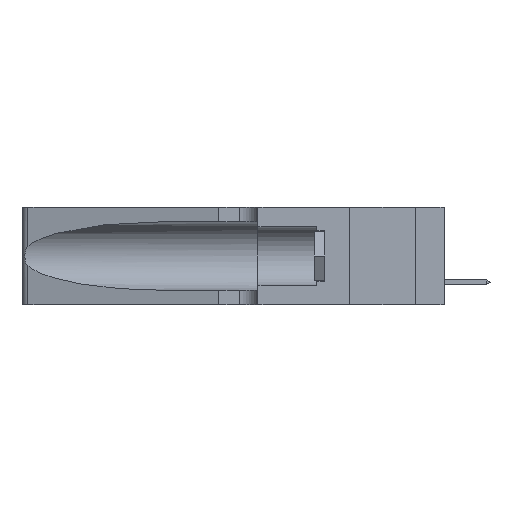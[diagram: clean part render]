
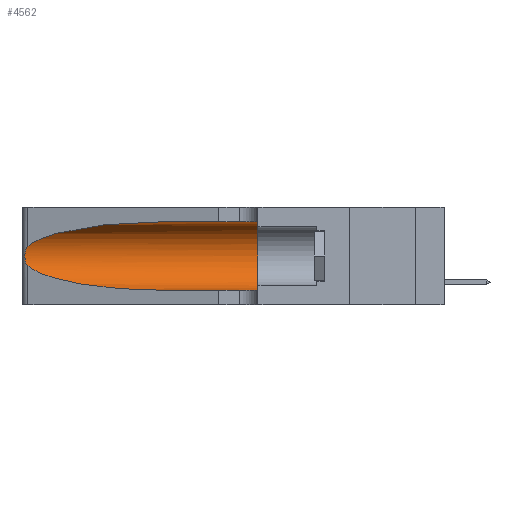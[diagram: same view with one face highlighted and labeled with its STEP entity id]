
A CAD part, left-side view. The second image highlights one B-rep face of the part: STEP entity #4562.
In plain terms, the highlighted cylindrical face has radius 3.308 mm (diameter 6.617 mm), a partial arc.
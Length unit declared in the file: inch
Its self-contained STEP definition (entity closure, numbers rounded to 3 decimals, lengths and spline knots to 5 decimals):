
#652 = ORIENTED_EDGE ( 'NONE', *, *, #2996, .T. ) ;
#732 = LINE ( 'NONE', #8319, #9041 ) ;
#810 = EDGE_CURVE ( 'NONE', #3578, #13876, #20713, .T. ) ;
#1320 = DIRECTION ( 'NONE',  ( 0., -1., 0. ) ) ;
#1376 = CARTESIAN_POINT ( 'NONE',  ( 0.25639, 1.23184, 0.21858 ) ) ;
#1530 = CARTESIAN_POINT ( 'NONE',  ( 0.25789, 1.23486, 0.15765 ) ) ;
#2424 =( BOUNDED_CURVE ( )  B_SPLINE_CURVE ( 3, ( #16132, #9029, #17956, #18024 ),
 .UNSPECIFIED., .F., .F. ) 
 B_SPLINE_CURVE_WITH_KNOTS ( ( 4, 4 ),
 ( 3.44316, 4.71239 ),
 .UNSPECIFIED. ) 
 CURVE ( )  GEOMETRIC_REPRESENTATION_ITEM ( )  RATIONAL_B_SPLINE_CURVE ( ( 1., 0.87, 0.87, 1. ) ) 
 REPRESENTATION_ITEM ( '' )  );
#2996 = EDGE_CURVE ( 'NONE', #15534, #13876, #9324, .T. ) ;
#3229 = CARTESIAN_POINT ( 'NONE',  ( 0.25854, 1.2359, 0.20912 ) ) ;
#3366 = DIRECTION ( 'NONE',  ( 0., -1., 0. ) ) ;
#3578 = VERTEX_POINT ( 'NONE', #5472 ) ;
#4065 = CARTESIAN_POINT ( 'NONE',  ( 0.18966, 0.96281, 0.31525 ) ) ;
#4504 = VECTOR ( 'NONE', #1320, 39.37008 ) ;
#4562 = ADVANCED_FACE ( 'NONE', ( #17464 ), #7822, .F. ) ;
#4864 = EDGE_LOOP ( 'NONE', ( #17636, #15451, #6597, #652, #12323, #9043 ) ) ;
#4924 = CARTESIAN_POINT ( 'NONE',  ( 0.25487, 1.22718, 0.22369 ) ) ;
#5076 = CARTESIAN_POINT ( 'NONE',  ( 0.26075, 1.23896, 0.19203 ) ) ;
#5120 = DIRECTION ( 'NONE',  ( 0., 0., -1. ) ) ;
#5224 = CARTESIAN_POINT ( 'NONE',  ( 0.26018, 1.23835, 0.19895 ) ) ;
#5472 = CARTESIAN_POINT ( 'NONE',  ( 0.1305, 0.35, 0.31525 ) ) ;
#6391 = CARTESIAN_POINT ( 'NONE',  ( 0.1305, 0.72297, 0.05475 ) ) ;
#6597 = ORIENTED_EDGE ( 'NONE', *, *, #18914, .T. ) ;
#7049 = CARTESIAN_POINT ( 'NONE',  ( 0.1305, 1.61858, 0.185 ) ) ;
#7211 = VERTEX_POINT ( 'NONE', #11673 ) ;
#7288 = EDGE_CURVE ( 'NONE', #7211, #9156, #22799, .T. ) ;
#7822 = CYLINDRICAL_SURFACE ( 'NONE', #10028, 0.13025 ) ;
#8319 = CARTESIAN_POINT ( 'NONE',  ( 0.1305, 1.61858, 0.31525 ) ) ;
#8689 = CARTESIAN_POINT ( 'NONE',  ( 0.1305, 1.61858, 0.05475 ) ) ;
#8825 = EDGE_CURVE ( 'NONE', #7211, #3578, #732, .T. ) ;
#8898 = VERTEX_POINT ( 'NONE', #14231 ) ;
#9029 = CARTESIAN_POINT ( 'NONE',  ( 0.2373, 1.15595, 0.08982 ) ) ;
#9041 = VECTOR ( 'NONE', #10214, 39.37008 ) ;
#9043 = ORIENTED_EDGE ( 'NONE', *, *, #8825, .F. ) ;
#9156 = VERTEX_POINT ( 'NONE', #12127 ) ;
#9324 = LINE ( 'NONE', #8689, #4504 ) ;
#9572 = B_SPLINE_CURVE_WITH_KNOTS ( 'NONE', 3,
 ( #4924, #21310, #1376, #14080, #3229, #5224, #5076, #15909, #17897, #14166, #1530, #14998, #17075, #12709 ),
 .UNSPECIFIED., .F., .F.,
 ( 4, 2, 2, 2, 2, 2, 4 ),
 ( 0., 0.00027, 0.00053, 0.00107, 0.0016, 0.00187, 0.00214 ),
 .UNSPECIFIED. ) ;
#9988 = CARTESIAN_POINT ( 'NONE',  ( 0.1305, 0.35, 0.05475 ) ) ;
#10028 = AXIS2_PLACEMENT_3D ( 'NONE', #7049, #3366, #5120 ) ;
#10214 = DIRECTION ( 'NONE',  ( 0., -1., 0. ) ) ;
#10272 = DIRECTION ( 'NONE',  ( 0., 0., 1. ) ) ;
#11206 = CARTESIAN_POINT ( 'NONE',  ( 0.2373, 1.15595, 0.28018 ) ) ;
#11673 = CARTESIAN_POINT ( 'NONE',  ( 0.1305, 0.72297, 0.31525 ) ) ;
#12127 = CARTESIAN_POINT ( 'NONE',  ( 0.25487, 1.22718, 0.22369 ) ) ;
#12323 = ORIENTED_EDGE ( 'NONE', *, *, #810, .F. ) ;
#12709 = CARTESIAN_POINT ( 'NONE',  ( 0.25487, 1.22718, 0.14631 ) ) ;
#13876 = VERTEX_POINT ( 'NONE', #9988 ) ;
#14080 = CARTESIAN_POINT ( 'NONE',  ( 0.25787, 1.23484, 0.2124 ) ) ;
#14166 = CARTESIAN_POINT ( 'NONE',  ( 0.25856, 1.23593, 0.16098 ) ) ;
#14231 = CARTESIAN_POINT ( 'NONE',  ( 0.25487, 1.22718, 0.14631 ) ) ;
#14998 = CARTESIAN_POINT ( 'NONE',  ( 0.25639, 1.23186, 0.15144 ) ) ;
#15451 = ORIENTED_EDGE ( 'NONE', *, *, #17910, .T. ) ;
#15534 = VERTEX_POINT ( 'NONE', #6391 ) ;
#15909 = CARTESIAN_POINT ( 'NONE',  ( 0.26075, 1.23896, 0.178 ) ) ;
#16132 = CARTESIAN_POINT ( 'NONE',  ( 0.25487, 1.22718, 0.14631 ) ) ;
#17075 = CARTESIAN_POINT ( 'NONE',  ( 0.25555, 1.22993, 0.14849 ) ) ;
#17464 = FACE_OUTER_BOUND ( 'NONE', #4864, .T. ) ;
#17636 = ORIENTED_EDGE ( 'NONE', *, *, #7288, .T. ) ;
#17897 = CARTESIAN_POINT ( 'NONE',  ( 0.26017, 1.23833, 0.17102 ) ) ;
#17910 = EDGE_CURVE ( 'NONE', #9156, #8898, #9572, .T. ) ;
#17956 = CARTESIAN_POINT ( 'NONE',  ( 0.18966, 0.96281, 0.05475 ) ) ;
#17991 = AXIS2_PLACEMENT_3D ( 'NONE', #21132, #19394, #10272 ) ;
#18024 = CARTESIAN_POINT ( 'NONE',  ( 0.1305, 0.72297, 0.05475 ) ) ;
#18734 = CARTESIAN_POINT ( 'NONE',  ( 0.1305, 0.72297, 0.31525 ) ) ;
#18914 = EDGE_CURVE ( 'NONE', #8898, #15534, #2424, .T. ) ;
#19394 = DIRECTION ( 'NONE',  ( 0., 1., 0. ) ) ;
#20253 = CARTESIAN_POINT ( 'NONE',  ( 0.25487, 1.22718, 0.22369 ) ) ;
#20713 = CIRCLE ( 'NONE', #17991, 0.13025 ) ;
#21132 = CARTESIAN_POINT ( 'NONE',  ( 0.1305, 0.35, 0.185 ) ) ;
#21310 = CARTESIAN_POINT ( 'NONE',  ( 0.25555, 1.22994, 0.2215 ) ) ;
#22799 =( BOUNDED_CURVE ( )  B_SPLINE_CURVE ( 3, ( #18734, #4065, #11206, #20253 ),
 .UNSPECIFIED., .F., .T. ) 
 B_SPLINE_CURVE_WITH_KNOTS ( ( 4, 4 ),
 ( 1.5708, 2.84003 ),
 .UNSPECIFIED. ) 
 CURVE ( )  GEOMETRIC_REPRESENTATION_ITEM ( )  RATIONAL_B_SPLINE_CURVE ( ( 1., 0.87, 0.87, 1. ) ) 
 REPRESENTATION_ITEM ( '' )  );
